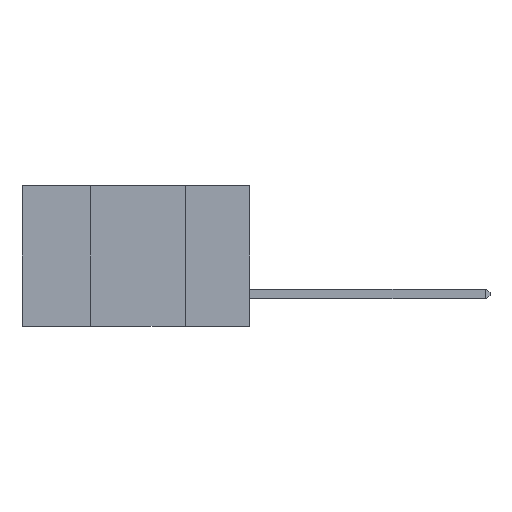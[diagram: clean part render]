
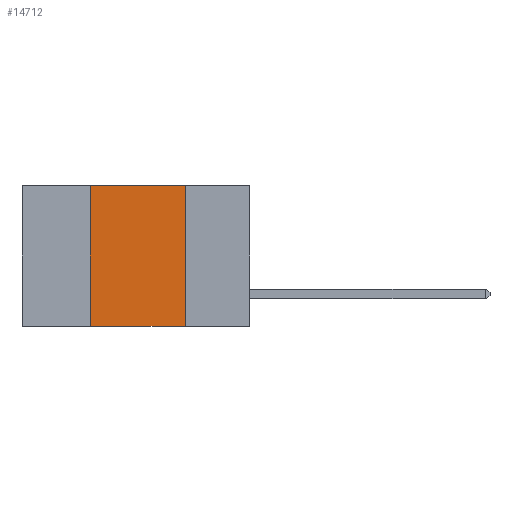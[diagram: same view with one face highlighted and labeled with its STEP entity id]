
A CAD part, left-side view. The second image highlights one B-rep face of the part: STEP entity #14712.
In plain terms, the highlighted planar face has unit normal (-1, 0, 0).
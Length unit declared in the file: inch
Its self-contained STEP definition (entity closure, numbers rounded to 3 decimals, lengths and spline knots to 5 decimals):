
#618 = VECTOR ( 'NONE', #2893, 39.37008 ) ;
#1220 = EDGE_CURVE ( 'NONE', #16483, #4795, #13694, .T. ) ;
#1472 = CARTESIAN_POINT ( 'NONE',  ( 0., 0.42, 0. ) ) ;
#1927 = ORIENTED_EDGE ( 'NONE', *, *, #1220, .F. ) ;
#2001 = CARTESIAN_POINT ( 'NONE',  ( 0., 0.17, 0. ) ) ;
#2118 = CARTESIAN_POINT ( 'NONE',  ( 0., 0.42, 0. ) ) ;
#2222 = CARTESIAN_POINT ( 'NONE',  ( 0., 0.6, 0. ) ) ;
#2893 = DIRECTION ( 'NONE',  ( 0., 0., 1. ) ) ;
#3620 = EDGE_CURVE ( 'NONE', #7933, #13724, #15094, .T. ) ;
#3932 = CARTESIAN_POINT ( 'NONE',  ( 0., 0.6, 0. ) ) ;
#4350 = ORIENTED_EDGE ( 'NONE', *, *, #3620, .F. ) ;
#4795 = VERTEX_POINT ( 'NONE', #11333 ) ;
#4851 = DIRECTION ( 'NONE',  ( 0., -1., 0. ) ) ;
#6306 = AXIS2_PLACEMENT_3D ( 'NONE', #3932, #16559, #8209 ) ;
#6529 = ORIENTED_EDGE ( 'NONE', *, *, #17469, .F. ) ;
#6829 = PLANE ( 'NONE',  #6306 ) ;
#6956 = EDGE_CURVE ( 'NONE', #7933, #4795, #16939, .T. ) ;
#7933 = VERTEX_POINT ( 'NONE', #13943 ) ;
#8209 = DIRECTION ( 'NONE',  ( 0., 0., -1. ) ) ;
#8304 = ORIENTED_EDGE ( 'NONE', *, *, #6956, .T. ) ;
#8967 = CARTESIAN_POINT ( 'NONE',  ( 0., 0.6, -0.37 ) ) ;
#9967 = VECTOR ( 'NONE', #14645, 39.37008 ) ;
#10643 = DIRECTION ( 'NONE',  ( 0., -1., 0. ) ) ;
#11138 = VECTOR ( 'NONE', #10643, 39.37008 ) ;
#11333 = CARTESIAN_POINT ( 'NONE',  ( 0., 0.17, -0.37 ) ) ;
#13228 = VECTOR ( 'NONE', #4851, 39.37008 ) ;
#13694 = LINE ( 'NONE', #2001, #9967 ) ;
#13724 = VERTEX_POINT ( 'NONE', #2118 ) ;
#13943 = CARTESIAN_POINT ( 'NONE',  ( 0., 0.42, -0.37 ) ) ;
#14645 = DIRECTION ( 'NONE',  ( 0., 0., -1. ) ) ;
#14712 = ADVANCED_FACE ( 'NONE', ( #17541 ), #6829, .F. ) ;
#14751 = EDGE_LOOP ( 'NONE', ( #1927, #6529, #4350, #8304 ) ) ;
#14833 = CARTESIAN_POINT ( 'NONE',  ( 0., 0.17, 0. ) ) ;
#15094 = LINE ( 'NONE', #1472, #618 ) ;
#15295 = LINE ( 'NONE', #2222, #11138 ) ;
#16483 = VERTEX_POINT ( 'NONE', #14833 ) ;
#16559 = DIRECTION ( 'NONE',  ( 1., 0., 0. ) ) ;
#16939 = LINE ( 'NONE', #8967, #13228 ) ;
#17469 = EDGE_CURVE ( 'NONE', #13724, #16483, #15295, .T. ) ;
#17541 = FACE_OUTER_BOUND ( 'NONE', #14751, .T. ) ;
